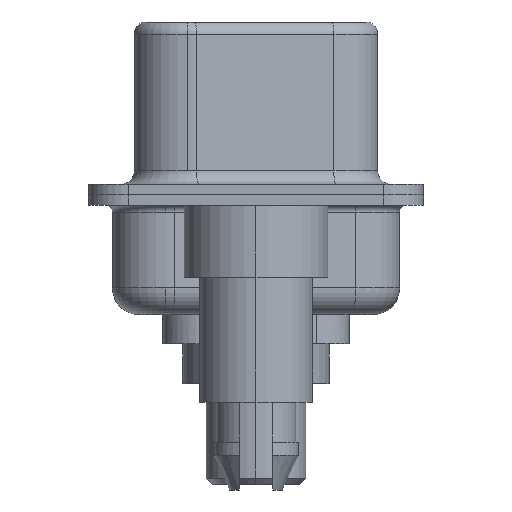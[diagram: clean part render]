
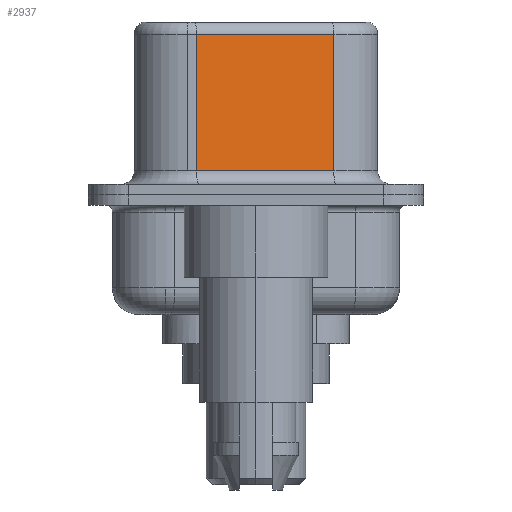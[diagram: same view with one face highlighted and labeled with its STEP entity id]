
A CAD part, left-side view. The second image highlights one B-rep face of the part: STEP entity #2937.
In plain terms, the highlighted planar face has unit normal (-0.985, -0.174, 0).
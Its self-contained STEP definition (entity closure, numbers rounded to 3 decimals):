
#260 = VERTEX_POINT ( 'NONE', #5928 ) ;
#732 = DIRECTION ( 'NONE',  ( -0.174, 0.985, 0. ) ) ;
#749 = DIRECTION ( 'NONE',  ( 0.985, 0.174, 0. ) ) ;
#1219 = VECTOR ( 'NONE', #5022, 1000. ) ;
#1295 = ORIENTED_EDGE ( 'NONE', *, *, #4169, .F. ) ;
#1611 = LINE ( 'NONE', #10801, #1219 ) ;
#2936 = EDGE_CURVE ( 'NONE', #260, #14995, #14812, .T. ) ;
#2937 = ADVANCED_FACE ( 'NONE', ( #8479 ), #13596, .F. ) ;
#3115 = VECTOR ( 'NONE', #7075, 1000. ) ;
#3353 = CARTESIAN_POINT ( 'NONE',  ( 4.58, -2.927, 6.02 ) ) ;
#3435 = VERTEX_POINT ( 'NONE', #3353 ) ;
#4011 = VERTEX_POINT ( 'NONE', #5145 ) ;
#4169 = EDGE_CURVE ( 'NONE', #3435, #4011, #9330, .T. ) ;
#4332 = EDGE_CURVE ( 'NONE', #14995, #4011, #13538, .T. ) ;
#5022 = DIRECTION ( 'NONE',  ( -0.174, 0.985, 0. ) ) ;
#5145 = CARTESIAN_POINT ( 'NONE',  ( 4.58, -2.927, 0.9 ) ) ;
#5928 = CARTESIAN_POINT ( 'NONE',  ( 3.67, 2.233, 6.02 ) ) ;
#6440 = CARTESIAN_POINT ( 'NONE',  ( 4.58, -2.927, 6.52 ) ) ;
#7075 = DIRECTION ( 'NONE',  ( 0., 0., -1. ) ) ;
#7215 = VECTOR ( 'NONE', #8226, 1000. ) ;
#8226 = DIRECTION ( 'NONE',  ( 0.174, -0.985, 0. ) ) ;
#8479 = FACE_OUTER_BOUND ( 'NONE', #14732, .T. ) ;
#8815 = VECTOR ( 'NONE', #10232, 1000. ) ;
#9330 = LINE ( 'NONE', #14389, #3115 ) ;
#10232 = DIRECTION ( 'NONE',  ( 0., 0., -1. ) ) ;
#10801 = CARTESIAN_POINT ( 'NONE',  ( 4.58, -2.927, 6.02 ) ) ;
#11412 = CARTESIAN_POINT ( 'NONE',  ( 3.67, 2.233, 6.52 ) ) ;
#11762 = EDGE_CURVE ( 'NONE', #3435, #260, #1611, .T. ) ;
#12540 = CARTESIAN_POINT ( 'NONE',  ( 3.67, 2.233, 0.9 ) ) ;
#13538 = LINE ( 'NONE', #13739, #7215 ) ;
#13596 = PLANE ( 'NONE',  #13692 ) ;
#13692 = AXIS2_PLACEMENT_3D ( 'NONE', #6440, #749, #732 ) ;
#13739 = CARTESIAN_POINT ( 'NONE',  ( 4.58, -2.927, 0.9 ) ) ;
#14021 = ORIENTED_EDGE ( 'NONE', *, *, #11762, .T. ) ;
#14389 = CARTESIAN_POINT ( 'NONE',  ( 4.58, -2.927, 6.52 ) ) ;
#14639 = ORIENTED_EDGE ( 'NONE', *, *, #4332, .T. ) ;
#14717 = ORIENTED_EDGE ( 'NONE', *, *, #2936, .T. ) ;
#14732 = EDGE_LOOP ( 'NONE', ( #1295, #14021, #14717, #14639 ) ) ;
#14812 = LINE ( 'NONE', #11412, #8815 ) ;
#14995 = VERTEX_POINT ( 'NONE', #12540 ) ;
